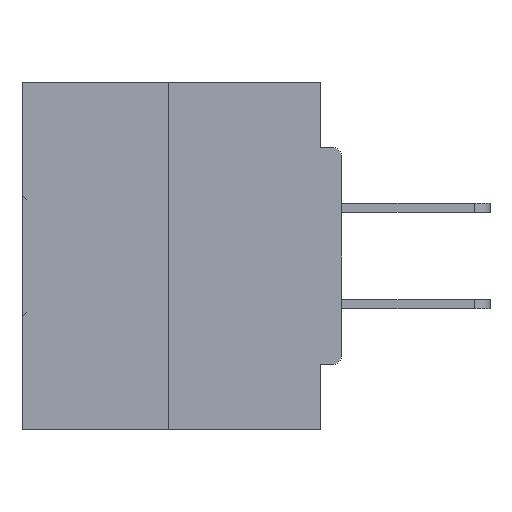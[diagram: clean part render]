
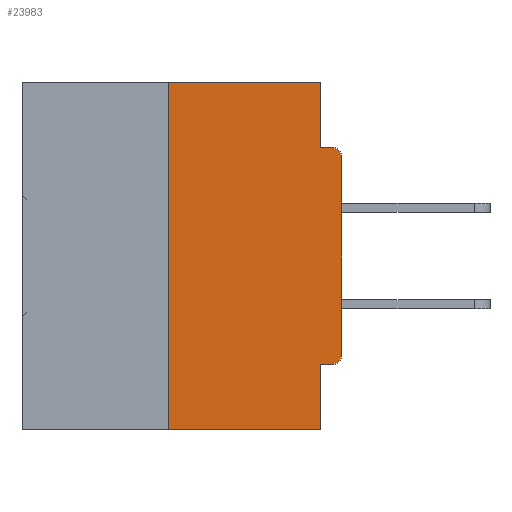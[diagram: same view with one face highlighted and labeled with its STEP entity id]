
A CAD part, left-side view. The second image highlights one B-rep face of the part: STEP entity #23983.
In plain terms, the highlighted planar face has unit normal (-1, 0, 0).
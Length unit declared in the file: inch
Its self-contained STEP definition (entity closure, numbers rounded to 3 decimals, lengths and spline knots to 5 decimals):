
#151 = DIRECTION ( 'NONE',  ( 0., -1., 0. ) ) ;
#165 = AXIS2_PLACEMENT_3D ( 'NONE', #19138, #37204, #11477 ) ;
#456 = EDGE_CURVE ( 'NONE', #11185, #16312, #23088, .T. ) ;
#918 = CARTESIAN_POINT ( 'NONE',  ( 0., 0.46, 0. ) ) ;
#2336 = CARTESIAN_POINT ( 'NONE',  ( 0., 0.015, -0.1085 ) ) ;
#2420 = EDGE_CURVE ( 'NONE', #35765, #16312, #17833, .T. ) ;
#2731 = DIRECTION ( 'NONE',  ( 0., 0., 1. ) ) ;
#3491 = CARTESIAN_POINT ( 'NONE',  ( 0., 0.46, -0.5 ) ) ;
#3601 = CARTESIAN_POINT ( 'NONE',  ( 0., 0., -0.1085 ) ) ;
#3938 = AXIS2_PLACEMENT_3D ( 'NONE', #2336, #9762, #45690 ) ;
#5299 = VERTEX_POINT ( 'NONE', #21413 ) ;
#5787 = DIRECTION ( 'NONE',  ( 0., 0., -1. ) ) ;
#6064 = CARTESIAN_POINT ( 'NONE',  ( 0., 0., 0. ) ) ;
#8056 = LINE ( 'NONE', #918, #40009 ) ;
#8315 = VERTEX_POINT ( 'NONE', #25189 ) ;
#9073 = FACE_OUTER_BOUND ( 'NONE', #28682, .T. ) ;
#9075 = EDGE_CURVE ( 'NONE', #8315, #12046, #27715, .T. ) ;
#9762 = DIRECTION ( 'NONE',  ( -1., 0., 0. ) ) ;
#11141 = ORIENTED_EDGE ( 'NONE', *, *, #42197, .F. ) ;
#11185 = VERTEX_POINT ( 'NONE', #3601 ) ;
#11477 = DIRECTION ( 'NONE',  ( 0., 0., -1. ) ) ;
#11722 = ORIENTED_EDGE ( 'NONE', *, *, #9075, .T. ) ;
#11788 = PLANE ( 'NONE',  #165 ) ;
#11845 = LINE ( 'NONE', #6064, #29161 ) ;
#12046 = VERTEX_POINT ( 'NONE', #21063 ) ;
#12080 = DIRECTION ( 'NONE',  ( 0., 0., 1. ) ) ;
#12089 = AXIS2_PLACEMENT_3D ( 'NONE', #17386, #27889, #38873 ) ;
#14339 = LINE ( 'NONE', #34040, #41885 ) ;
#14579 = VECTOR ( 'NONE', #45881, 39.37008 ) ;
#15701 = CARTESIAN_POINT ( 'NONE',  ( 0., 0., -0.3915 ) ) ;
#15732 = DIRECTION ( 'NONE',  ( 0., -1., 0. ) ) ;
#16312 = VERTEX_POINT ( 'NONE', #25640 ) ;
#16501 = ORIENTED_EDGE ( 'NONE', *, *, #456, .T. ) ;
#17005 = EDGE_CURVE ( 'NONE', #27640, #40594, #20571, .T. ) ;
#17147 = CARTESIAN_POINT ( 'NONE',  ( 0., 0., -0.4065 ) ) ;
#17386 = CARTESIAN_POINT ( 'NONE',  ( 0., 0.015, -0.3915 ) ) ;
#17833 = LINE ( 'NONE', #44101, #45372 ) ;
#17894 = VERTEX_POINT ( 'NONE', #21247 ) ;
#19138 = CARTESIAN_POINT ( 'NONE',  ( 0., 0.46, 0. ) ) ;
#19438 = CARTESIAN_POINT ( 'NONE',  ( 0., 0.015, -0.4065 ) ) ;
#20066 = CARTESIAN_POINT ( 'NONE',  ( 0., 0.031, -0.5 ) ) ;
#20571 = CIRCLE ( 'NONE', #12089, 0.015 ) ;
#21063 = CARTESIAN_POINT ( 'NONE',  ( 0., 0.031, -0.5 ) ) ;
#21247 = CARTESIAN_POINT ( 'NONE',  ( 0., 0.25, 0. ) ) ;
#21413 = CARTESIAN_POINT ( 'NONE',  ( 0., 0.031, -0.4065 ) ) ;
#22914 = DIRECTION ( 'NONE',  ( 0., -1., 0. ) ) ;
#22970 = EDGE_CURVE ( 'NONE', #5299, #12046, #31642, .T. ) ;
#23088 = CIRCLE ( 'NONE', #3938, 0.015 ) ;
#23862 = CARTESIAN_POINT ( 'NONE',  ( 0., 0.031, 0. ) ) ;
#23983 = ADVANCED_FACE ( 'NONE', ( #9073 ), #11788, .F. ) ;
#24785 = ORIENTED_EDGE ( 'NONE', *, *, #45631, .F. ) ;
#25189 = CARTESIAN_POINT ( 'NONE',  ( 0., 0.25, -0.5 ) ) ;
#25640 = CARTESIAN_POINT ( 'NONE',  ( 0., 0.015, -0.0935 ) ) ;
#25951 = ORIENTED_EDGE ( 'NONE', *, *, #17005, .T. ) ;
#27027 = VERTEX_POINT ( 'NONE', #39944 ) ;
#27411 = ORIENTED_EDGE ( 'NONE', *, *, #2420, .F. ) ;
#27640 = VERTEX_POINT ( 'NONE', #19438 ) ;
#27715 = LINE ( 'NONE', #3491, #29359 ) ;
#27805 = VECTOR ( 'NONE', #40421, 39.37008 ) ;
#27889 = DIRECTION ( 'NONE',  ( -1., 0., 0. ) ) ;
#28212 = VECTOR ( 'NONE', #5787, 39.37008 ) ;
#28348 = ORIENTED_EDGE ( 'NONE', *, *, #42059, .F. ) ;
#28682 = EDGE_LOOP ( 'NONE', ( #34838, #11141, #11722, #30848, #24785, #25951, #30278, #16501, #27411, #28348 ) ) ;
#29161 = VECTOR ( 'NONE', #2731, 39.37008 ) ;
#29359 = VECTOR ( 'NONE', #151, 39.37008 ) ;
#30278 = ORIENTED_EDGE ( 'NONE', *, *, #32968, .T. ) ;
#30848 = ORIENTED_EDGE ( 'NONE', *, *, #22970, .F. ) ;
#31403 = LINE ( 'NONE', #17147, #14579 ) ;
#31642 = LINE ( 'NONE', #20066, #28212 ) ;
#32968 = EDGE_CURVE ( 'NONE', #40594, #11185, #11845, .T. ) ;
#34040 = CARTESIAN_POINT ( 'NONE',  ( 0., 0.25, 0. ) ) ;
#34838 = ORIENTED_EDGE ( 'NONE', *, *, #36199, .F. ) ;
#35765 = VERTEX_POINT ( 'NONE', #37002 ) ;
#36199 = EDGE_CURVE ( 'NONE', #17894, #27027, #8056, .T. ) ;
#37002 = CARTESIAN_POINT ( 'NONE',  ( 0., 0.031, -0.0935 ) ) ;
#37204 = DIRECTION ( 'NONE',  ( 1., 0., 0. ) ) ;
#37383 = LINE ( 'NONE', #23862, #27805 ) ;
#38873 = DIRECTION ( 'NONE',  ( 0., 0., -1. ) ) ;
#39944 = CARTESIAN_POINT ( 'NONE',  ( 0., 0.031, 0. ) ) ;
#40009 = VECTOR ( 'NONE', #15732, 39.37008 ) ;
#40421 = DIRECTION ( 'NONE',  ( 0., 0., -1. ) ) ;
#40594 = VERTEX_POINT ( 'NONE', #15701 ) ;
#41885 = VECTOR ( 'NONE', #12080, 39.37008 ) ;
#42059 = EDGE_CURVE ( 'NONE', #27027, #35765, #37383, .T. ) ;
#42197 = EDGE_CURVE ( 'NONE', #8315, #17894, #14339, .T. ) ;
#44101 = CARTESIAN_POINT ( 'NONE',  ( 0., 0., -0.0935 ) ) ;
#45372 = VECTOR ( 'NONE', #22914, 39.37008 ) ;
#45631 = EDGE_CURVE ( 'NONE', #27640, #5299, #31403, .T. ) ;
#45690 = DIRECTION ( 'NONE',  ( 0., 0., -1. ) ) ;
#45881 = DIRECTION ( 'NONE',  ( 0., 1., 0. ) ) ;
